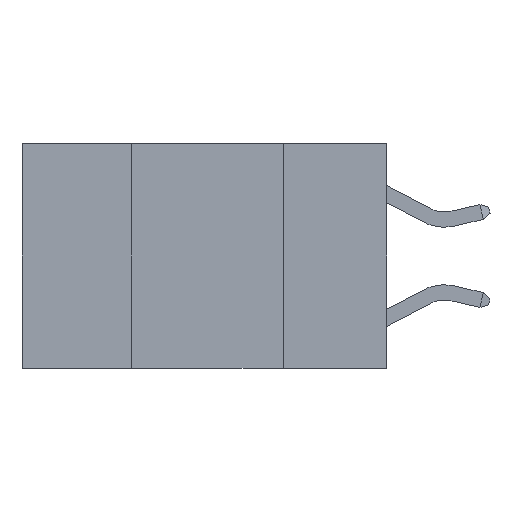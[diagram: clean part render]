
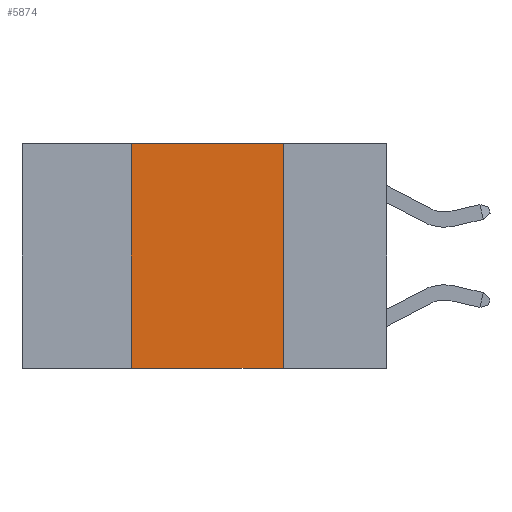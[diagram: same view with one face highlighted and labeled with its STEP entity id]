
A CAD part, left-side view. The second image highlights one B-rep face of the part: STEP entity #5874.
In plain terms, the highlighted planar face has unit normal (-1, 0, 0).
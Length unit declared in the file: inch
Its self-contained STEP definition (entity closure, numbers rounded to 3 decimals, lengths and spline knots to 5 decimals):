
#187 = PLANE ( 'NONE',  #9352 ) ;
#593 = VECTOR ( 'NONE', #1289, 39.37008 ) ;
#1258 = ORIENTED_EDGE ( 'NONE', *, *, #5677, .F. ) ;
#1289 = DIRECTION ( 'NONE',  ( 0., -1., 0. ) ) ;
#1589 = CARTESIAN_POINT ( 'NONE',  ( 0., 0.6, -0.37 ) ) ;
#1984 = CARTESIAN_POINT ( 'NONE',  ( 0., 0.42, 0. ) ) ;
#2116 = ORIENTED_EDGE ( 'NONE', *, *, #4262, .F. ) ;
#2119 = VERTEX_POINT ( 'NONE', #4790 ) ;
#2120 = DIRECTION ( 'NONE',  ( 0., 0., -1. ) ) ;
#2362 = VERTEX_POINT ( 'NONE', #6888 ) ;
#2587 = VERTEX_POINT ( 'NONE', #4267 ) ;
#2862 = CARTESIAN_POINT ( 'NONE',  ( 0., 0.6, 0. ) ) ;
#3011 = DIRECTION ( 'NONE',  ( 1., 0., 0. ) ) ;
#3198 = VECTOR ( 'NONE', #8279, 39.37008 ) ;
#3859 = EDGE_CURVE ( 'NONE', #2119, #2362, #9160, .T. ) ;
#3879 = VECTOR ( 'NONE', #9454, 39.37008 ) ;
#4262 = EDGE_CURVE ( 'NONE', #2119, #8246, #7314, .T. ) ;
#4267 = CARTESIAN_POINT ( 'NONE',  ( 0., 0.17, 0. ) ) ;
#4722 = LINE ( 'NONE', #2862, #593 ) ;
#4790 = CARTESIAN_POINT ( 'NONE',  ( 0., 0.42, -0.37 ) ) ;
#5677 = EDGE_CURVE ( 'NONE', #8246, #2587, #4722, .T. ) ;
#5841 = CARTESIAN_POINT ( 'NONE',  ( 0., 0.17, 0. ) ) ;
#5874 = ADVANCED_FACE ( 'NONE', ( #8340 ), #187, .F. ) ;
#6156 = CARTESIAN_POINT ( 'NONE',  ( 0., 0.6, 0. ) ) ;
#6888 = CARTESIAN_POINT ( 'NONE',  ( 0., 0.17, -0.37 ) ) ;
#7077 = EDGE_LOOP ( 'NONE', ( #8378, #1258, #2116, #8532 ) ) ;
#7314 = LINE ( 'NONE', #1984, #3879 ) ;
#7445 = EDGE_CURVE ( 'NONE', #2587, #2362, #8226, .T. ) ;
#7616 = CARTESIAN_POINT ( 'NONE',  ( 0., 0.42, 0. ) ) ;
#8226 = LINE ( 'NONE', #5841, #9173 ) ;
#8246 = VERTEX_POINT ( 'NONE', #7616 ) ;
#8279 = DIRECTION ( 'NONE',  ( 0., -1., 0. ) ) ;
#8340 = FACE_OUTER_BOUND ( 'NONE', #7077, .T. ) ;
#8378 = ORIENTED_EDGE ( 'NONE', *, *, #7445, .F. ) ;
#8532 = ORIENTED_EDGE ( 'NONE', *, *, #3859, .T. ) ;
#9160 = LINE ( 'NONE', #1589, #3198 ) ;
#9173 = VECTOR ( 'NONE', #2120, 39.37008 ) ;
#9352 = AXIS2_PLACEMENT_3D ( 'NONE', #6156, #3011, #9364 ) ;
#9364 = DIRECTION ( 'NONE',  ( 0., 0., -1. ) ) ;
#9454 = DIRECTION ( 'NONE',  ( 0., 0., 1. ) ) ;
